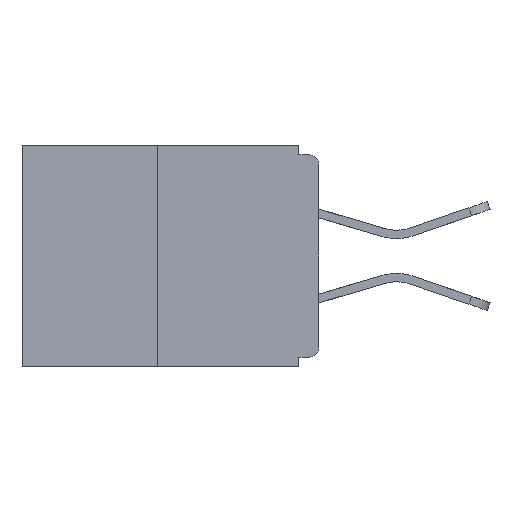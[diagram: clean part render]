
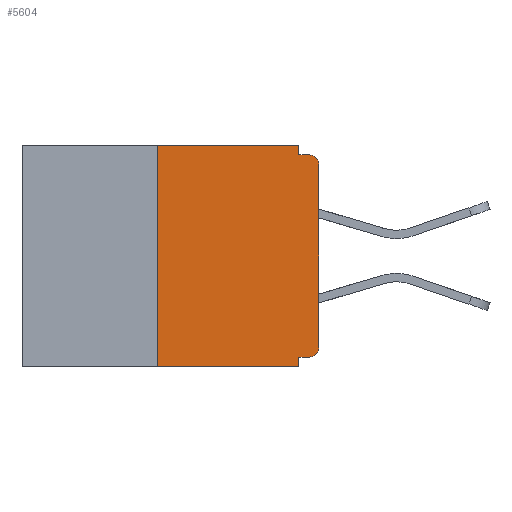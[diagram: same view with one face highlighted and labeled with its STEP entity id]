
A CAD part, left-side view. The second image highlights one B-rep face of the part: STEP entity #5604.
In plain terms, the highlighted planar face has unit normal (-1, 0, 0).
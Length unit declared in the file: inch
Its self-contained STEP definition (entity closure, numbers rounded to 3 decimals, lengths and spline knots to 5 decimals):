
#82 = AXIS2_PLACEMENT_3D ( 'NONE', #3760, #17980, #17918 ) ;
#327 = LINE ( 'NONE', #12521, #2745 ) ;
#334 = CARTESIAN_POINT ( 'NONE',  ( 0., 0.015, -0.313 ) ) ;
#392 = EDGE_CURVE ( 'NONE', #8036, #980, #1380, .T. ) ;
#430 = CARTESIAN_POINT ( 'NONE',  ( 0., 0.031, -0.328 ) ) ;
#530 = VECTOR ( 'NONE', #10001, 39.37008 ) ;
#619 = VECTOR ( 'NONE', #4332, 39.37008 ) ;
#980 = VERTEX_POINT ( 'NONE', #5669 ) ;
#1223 = CARTESIAN_POINT ( 'NONE',  ( 0., 0.015, -0.03 ) ) ;
#1380 = LINE ( 'NONE', #5991, #15662 ) ;
#1600 = DIRECTION ( 'NONE',  ( 0., 0., 1. ) ) ;
#1660 = CARTESIAN_POINT ( 'NONE',  ( 0., 0., -0.015 ) ) ;
#1721 = EDGE_LOOP ( 'NONE', ( #13857, #11767, #8310, #6120, #3077, #9350, #5184, #12491, #8518, #11179 ) ) ;
#1885 = DIRECTION ( 'NONE',  ( 0., 0., -1. ) ) ;
#1930 = FACE_OUTER_BOUND ( 'NONE', #1721, .T. ) ;
#2718 = DIRECTION ( 'NONE',  ( 0., 0., -1. ) ) ;
#2745 = VECTOR ( 'NONE', #15170, 39.37008 ) ;
#3077 = ORIENTED_EDGE ( 'NONE', *, *, #13192, .F. ) ;
#3226 = CARTESIAN_POINT ( 'NONE',  ( 0., 0.031, -0.343 ) ) ;
#3760 = CARTESIAN_POINT ( 'NONE',  ( 0., 0.46, 0. ) ) ;
#4157 = LINE ( 'NONE', #13063, #17557 ) ;
#4167 = AXIS2_PLACEMENT_3D ( 'NONE', #334, #4889, #1885 ) ;
#4332 = DIRECTION ( 'NONE',  ( 0., 0., -1. ) ) ;
#4656 = DIRECTION ( 'NONE',  ( 0., 0., -1. ) ) ;
#4825 = VERTEX_POINT ( 'NONE', #11659 ) ;
#4889 = DIRECTION ( 'NONE',  ( -1., 0., 0. ) ) ;
#5064 = LINE ( 'NONE', #8597, #619 ) ;
#5182 = VECTOR ( 'NONE', #7885, 39.37008 ) ;
#5184 = ORIENTED_EDGE ( 'NONE', *, *, #392, .T. ) ;
#5604 = ADVANCED_FACE ( 'NONE', ( #1930 ), #13598, .F. ) ;
#5669 = CARTESIAN_POINT ( 'NONE',  ( 0., 0., -0.03 ) ) ;
#5991 = CARTESIAN_POINT ( 'NONE',  ( 0., 0., 0. ) ) ;
#6120 = ORIENTED_EDGE ( 'NONE', *, *, #12966, .F. ) ;
#6344 = CIRCLE ( 'NONE', #4167, 0.015 ) ;
#6345 = CARTESIAN_POINT ( 'NONE',  ( 0., 0.031, -0.343 ) ) ;
#7865 = VERTEX_POINT ( 'NONE', #6345 ) ;
#7885 = DIRECTION ( 'NONE',  ( 0., -1., 0. ) ) ;
#8036 = VERTEX_POINT ( 'NONE', #8834 ) ;
#8310 = ORIENTED_EDGE ( 'NONE', *, *, #15139, .T. ) ;
#8326 = EDGE_CURVE ( 'NONE', #4825, #8036, #6344, .T. ) ;
#8518 = ORIENTED_EDGE ( 'NONE', *, *, #15882, .F. ) ;
#8597 = CARTESIAN_POINT ( 'NONE',  ( 0., 0.031, 0. ) ) ;
#8825 = VERTEX_POINT ( 'NONE', #17373 ) ;
#8834 = CARTESIAN_POINT ( 'NONE',  ( 0., 0., -0.313 ) ) ;
#8985 = LINE ( 'NONE', #13446, #5182 ) ;
#9350 = ORIENTED_EDGE ( 'NONE', *, *, #8326, .T. ) ;
#9768 = EDGE_CURVE ( 'NONE', #13843, #16319, #8985, .T. ) ;
#9824 = EDGE_CURVE ( 'NONE', #8825, #13843, #327, .T. ) ;
#10001 = DIRECTION ( 'NONE',  ( 0., -1., 0. ) ) ;
#10499 = VERTEX_POINT ( 'NONE', #16191 ) ;
#10782 = VECTOR ( 'NONE', #14717, 39.37008 ) ;
#10826 = AXIS2_PLACEMENT_3D ( 'NONE', #1223, #15689, #2718 ) ;
#10981 = LINE ( 'NONE', #1660, #530 ) ;
#11068 = CARTESIAN_POINT ( 'NONE',  ( 0., 0.015, -0.015 ) ) ;
#11179 = ORIENTED_EDGE ( 'NONE', *, *, #13591, .F. ) ;
#11659 = CARTESIAN_POINT ( 'NONE',  ( 0., 0.015, -0.328 ) ) ;
#11683 = VERTEX_POINT ( 'NONE', #11068 ) ;
#11767 = ORIENTED_EDGE ( 'NONE', *, *, #9824, .F. ) ;
#12491 = ORIENTED_EDGE ( 'NONE', *, *, #16597, .T. ) ;
#12521 = CARTESIAN_POINT ( 'NONE',  ( 0., 0.25, 0. ) ) ;
#12966 = EDGE_CURVE ( 'NONE', #18303, #7865, #16667, .T. ) ;
#13063 = CARTESIAN_POINT ( 'NONE',  ( 0., 0., -0.328 ) ) ;
#13192 = EDGE_CURVE ( 'NONE', #4825, #18303, #4157, .T. ) ;
#13446 = CARTESIAN_POINT ( 'NONE',  ( 0., 0.46, 0. ) ) ;
#13591 = EDGE_CURVE ( 'NONE', #16319, #10499, #5064, .T. ) ;
#13596 = CIRCLE ( 'NONE', #10826, 0.015 ) ;
#13598 = PLANE ( 'NONE',  #82 ) ;
#13843 = VERTEX_POINT ( 'NONE', #18368 ) ;
#13857 = ORIENTED_EDGE ( 'NONE', *, *, #9768, .F. ) ;
#14418 = VECTOR ( 'NONE', #4656, 39.37008 ) ;
#14717 = DIRECTION ( 'NONE',  ( 0., -1., 0. ) ) ;
#15139 = EDGE_CURVE ( 'NONE', #8825, #7865, #18373, .T. ) ;
#15170 = DIRECTION ( 'NONE',  ( 0., 0., 1. ) ) ;
#15662 = VECTOR ( 'NONE', #1600, 39.37008 ) ;
#15689 = DIRECTION ( 'NONE',  ( -1., 0., 0. ) ) ;
#15795 = CARTESIAN_POINT ( 'NONE',  ( 0., 0.031, 0. ) ) ;
#15882 = EDGE_CURVE ( 'NONE', #10499, #11683, #10981, .T. ) ;
#16191 = CARTESIAN_POINT ( 'NONE',  ( 0., 0.031, -0.015 ) ) ;
#16319 = VERTEX_POINT ( 'NONE', #15795 ) ;
#16597 = EDGE_CURVE ( 'NONE', #980, #11683, #13596, .T. ) ;
#16667 = LINE ( 'NONE', #3226, #14418 ) ;
#17373 = CARTESIAN_POINT ( 'NONE',  ( 0., 0.25, -0.343 ) ) ;
#17377 = DIRECTION ( 'NONE',  ( 0., 1., 0. ) ) ;
#17557 = VECTOR ( 'NONE', #17377, 39.37008 ) ;
#17643 = CARTESIAN_POINT ( 'NONE',  ( 0., 0.46, -0.343 ) ) ;
#17918 = DIRECTION ( 'NONE',  ( 0., 0., -1. ) ) ;
#17980 = DIRECTION ( 'NONE',  ( 1., 0., 0. ) ) ;
#18303 = VERTEX_POINT ( 'NONE', #430 ) ;
#18368 = CARTESIAN_POINT ( 'NONE',  ( 0., 0.25, 0. ) ) ;
#18373 = LINE ( 'NONE', #17643, #10782 ) ;
